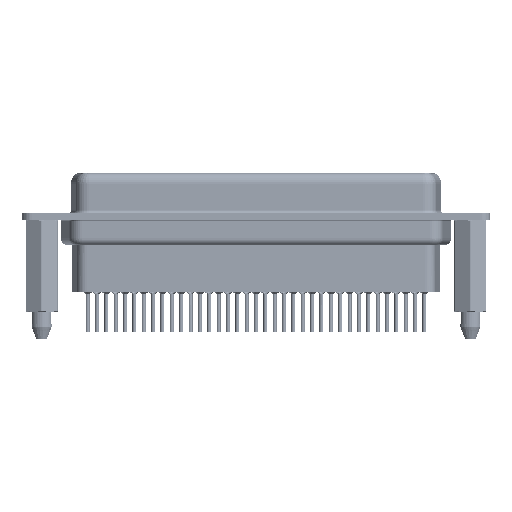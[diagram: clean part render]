
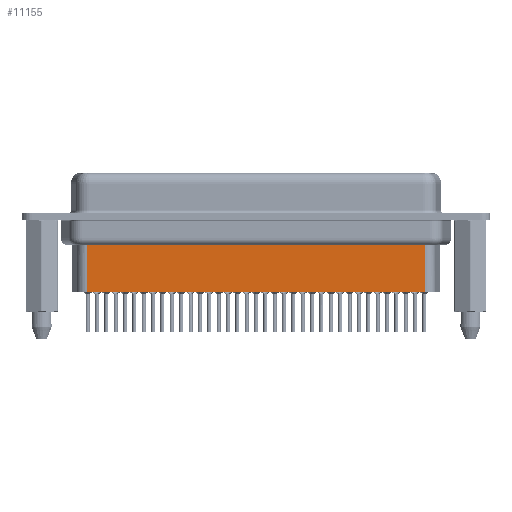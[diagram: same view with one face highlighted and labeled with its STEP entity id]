
A CAD part, front view. The second image highlights one B-rep face of the part: STEP entity #11155.
In plain terms, the highlighted planar face has unit normal (0, -1, 0).
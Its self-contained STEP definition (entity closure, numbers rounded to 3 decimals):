
#121 = DIRECTION ( 'NONE',  ( 0., -1., 0. ) ) ;
#1950 = CARTESIAN_POINT ( 'NONE',  ( 6.706, -3.5, -11.15 ) ) ;
#2545 = VECTOR ( 'NONE', #6859, 1000. ) ;
#3422 = VECTOR ( 'NONE', #6906, 1000. ) ;
#3457 = CARTESIAN_POINT ( 'NONE',  ( 6.459, -3.5, -4.097 ) ) ;
#3622 = DIRECTION ( 'NONE',  ( -1., 0., 0. ) ) ;
#6859 = DIRECTION ( 'NONE',  ( 0., 0., -1. ) ) ;
#6906 = DIRECTION ( 'NONE',  ( -1., 0., 0. ) ) ;
#9275 = LINE ( 'NONE', #27941, #2545 ) ;
#9672 = EDGE_CURVE ( 'NONE', #17470, #16335, #9275, .T. ) ;
#9842 = VERTEX_POINT ( 'NONE', #23985 ) ;
#10457 = VERTEX_POINT ( 'NONE', #29323 ) ;
#10580 = DIRECTION ( 'NONE',  ( 1., 0., 0. ) ) ;
#11011 = LINE ( 'NONE', #3457, #15993 ) ;
#11155 = ADVANCED_FACE ( 'NONE', ( #18450 ), #18960, .T. ) ;
#13412 = ORIENTED_EDGE ( 'NONE', *, *, #16170, .F. ) ;
#13987 = DIRECTION ( 'NONE',  ( 0., 0., -1. ) ) ;
#15993 = VECTOR ( 'NONE', #3622, 1000. ) ;
#16170 = EDGE_CURVE ( 'NONE', #16335, #10457, #28329, .T. ) ;
#16193 = CARTESIAN_POINT ( 'NONE',  ( 56.794, -3.5, -11.15 ) ) ;
#16335 = VERTEX_POINT ( 'NONE', #16193 ) ;
#16646 = ORIENTED_EDGE ( 'NONE', *, *, #31044, .T. ) ;
#17045 = VECTOR ( 'NONE', #13987, 1000. ) ;
#17470 = VERTEX_POINT ( 'NONE', #18811 ) ;
#18165 = ORIENTED_EDGE ( 'NONE', *, *, #28929, .T. ) ;
#18450 = FACE_OUTER_BOUND ( 'NONE', #19479, .T. ) ;
#18811 = CARTESIAN_POINT ( 'NONE',  ( 56.794, -3.5, -4.097 ) ) ;
#18960 = PLANE ( 'NONE',  #32836 ) ;
#19479 = EDGE_LOOP ( 'NONE', ( #27568, #16646, #18165, #13412 ) ) ;
#23578 = CARTESIAN_POINT ( 'NONE',  ( 6.706, -3.5, -3.1 ) ) ;
#23985 = CARTESIAN_POINT ( 'NONE',  ( 6.706, -3.5, -4.097 ) ) ;
#27568 = ORIENTED_EDGE ( 'NONE', *, *, #9672, .F. ) ;
#27941 = CARTESIAN_POINT ( 'NONE',  ( 56.794, -3.5, -3.1 ) ) ;
#28329 = LINE ( 'NONE', #1950, #3422 ) ;
#28929 = EDGE_CURVE ( 'NONE', #9842, #10457, #29566, .T. ) ;
#29323 = CARTESIAN_POINT ( 'NONE',  ( 6.706, -3.5, -11.15 ) ) ;
#29566 = LINE ( 'NONE', #32483, #17045 ) ;
#31044 = EDGE_CURVE ( 'NONE', #17470, #9842, #11011, .T. ) ;
#32483 = CARTESIAN_POINT ( 'NONE',  ( 6.706, -3.5, -3.1 ) ) ;
#32836 = AXIS2_PLACEMENT_3D ( 'NONE', #23578, #121, #10580 ) ;
